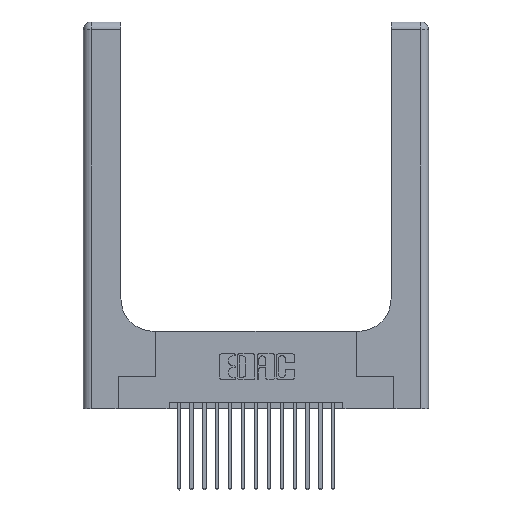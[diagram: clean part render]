
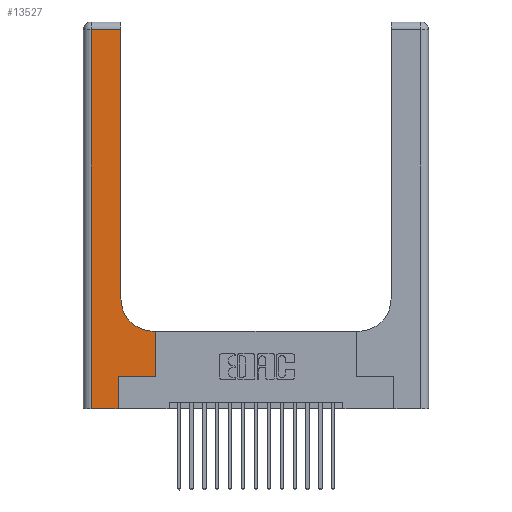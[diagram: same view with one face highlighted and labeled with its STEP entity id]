
A CAD part, top view. The second image highlights one B-rep face of the part: STEP entity #13527.
In plain terms, the highlighted planar face has unit normal (0, 0, 1).
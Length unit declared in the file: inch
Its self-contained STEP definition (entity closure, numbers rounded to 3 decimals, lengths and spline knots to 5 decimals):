
#70 = VERTEX_POINT ( 'NONE', #2962 ) ;
#95 = CARTESIAN_POINT ( 'NONE',  ( 0.06, 3., 0.37 ) ) ;
#214 = LINE ( 'NONE', #14687, #11632 ) ;
#369 = DIRECTION ( 'NONE',  ( 1., 0., 0. ) ) ;
#404 = FACE_OUTER_BOUND ( 'NONE', #9636, .T. ) ;
#464 = ORIENTED_EDGE ( 'NONE', *, *, #11493, .T. ) ;
#609 = VECTOR ( 'NONE', #3383, 39.37008 ) ;
#883 = VECTOR ( 'NONE', #18805, 39.37008 ) ;
#1662 = LINE ( 'NONE', #2473, #13062 ) ;
#1968 = EDGE_CURVE ( 'NONE', #17136, #9646, #12535, .T. ) ;
#2063 = PLANE ( 'NONE',  #4559 ) ;
#2333 = ORIENTED_EDGE ( 'NONE', *, *, #2672, .T. ) ;
#2473 = CARTESIAN_POINT ( 'NONE',  ( 0.2915, 0.6, 0.37 ) ) ;
#2625 = DIRECTION ( 'NONE',  ( 0., 1., 0. ) ) ;
#2672 = EDGE_CURVE ( 'NONE', #12663, #11301, #5974, .T. ) ;
#2962 = CARTESIAN_POINT ( 'NONE',  ( 0.06, 0., 0.37 ) ) ;
#3019 = LINE ( 'NONE', #15210, #12076 ) ;
#3383 = DIRECTION ( 'NONE',  ( 1., 0., 0. ) ) ;
#3759 = DIRECTION ( 'NONE',  ( 0., 0., -1. ) ) ;
#4023 = DIRECTION ( 'NONE',  ( -1., 0., 0. ) ) ;
#4559 = AXIS2_PLACEMENT_3D ( 'NONE', #5017, #3759, #6674 ) ;
#4581 = CARTESIAN_POINT ( 'NONE',  ( 0.269, 0., 0.37 ) ) ;
#4929 = VERTEX_POINT ( 'NONE', #9847 ) ;
#4987 = VERTEX_POINT ( 'NONE', #18731 ) ;
#5017 = CARTESIAN_POINT ( 'NONE',  ( 0., 3., 0.37 ) ) ;
#5289 = ORIENTED_EDGE ( 'NONE', *, *, #8573, .T. ) ;
#5542 = CARTESIAN_POINT ( 'NONE',  ( 0.2915, 3., 0.37 ) ) ;
#5974 = LINE ( 'NONE', #5542, #6220 ) ;
#6220 = VECTOR ( 'NONE', #13109, 39.37008 ) ;
#6235 = ORIENTED_EDGE ( 'NONE', *, *, #10613, .T. ) ;
#6674 = DIRECTION ( 'NONE',  ( -1., 0., 0. ) ) ;
#6829 = ORIENTED_EDGE ( 'NONE', *, *, #7333, .T. ) ;
#7162 = DIRECTION ( 'NONE',  ( 0., 0., -1. ) ) ;
#7333 = EDGE_CURVE ( 'NONE', #4987, #4929, #1662, .T. ) ;
#8206 = VERTEX_POINT ( 'NONE', #14205 ) ;
#8573 = EDGE_CURVE ( 'NONE', #70, #17136, #3019, .T. ) ;
#8642 = CIRCLE ( 'NONE', #11375, 0.25 ) ;
#8850 = EDGE_CURVE ( 'NONE', #9646, #8206, #16232, .T. ) ;
#8870 = CARTESIAN_POINT ( 'NONE',  ( 0.5415, 0.85, 0.37 ) ) ;
#9338 = VECTOR ( 'NONE', #11883, 39.37008 ) ;
#9636 = EDGE_LOOP ( 'NONE', ( #2333, #18656, #464, #5289, #10976, #10276, #15357, #6829, #6235 ) ) ;
#9646 = VERTEX_POINT ( 'NONE', #10710 ) ;
#9847 = CARTESIAN_POINT ( 'NONE',  ( 0.5415, 0.6, 0.37 ) ) ;
#10276 = ORIENTED_EDGE ( 'NONE', *, *, #8850, .T. ) ;
#10613 = EDGE_CURVE ( 'NONE', #4929, #12663, #8642, .T. ) ;
#10637 = CARTESIAN_POINT ( 'NONE',  ( 0.06, 2.94, 0.37 ) ) ;
#10710 = CARTESIAN_POINT ( 'NONE',  ( 0.269, 0.25, 0.37 ) ) ;
#10976 = ORIENTED_EDGE ( 'NONE', *, *, #1968, .T. ) ;
#11301 = VERTEX_POINT ( 'NONE', #18704 ) ;
#11346 = CARTESIAN_POINT ( 'NONE',  ( 0.269, 0., 0.37 ) ) ;
#11375 = AXIS2_PLACEMENT_3D ( 'NONE', #8870, #7162, #17603 ) ;
#11415 = EDGE_CURVE ( 'NONE', #11301, #17097, #214, .T. ) ;
#11493 = EDGE_CURVE ( 'NONE', #17097, #70, #11882, .T. ) ;
#11632 = VECTOR ( 'NONE', #16120, 39.37008 ) ;
#11643 = CARTESIAN_POINT ( 'NONE',  ( 0.2915, 0.85, 0.37 ) ) ;
#11882 = LINE ( 'NONE', #95, #9338 ) ;
#11883 = DIRECTION ( 'NONE',  ( 0., -1., 0. ) ) ;
#12022 = VECTOR ( 'NONE', #2625, 39.37008 ) ;
#12076 = VECTOR ( 'NONE', #369, 39.37008 ) ;
#12535 = LINE ( 'NONE', #11346, #883 ) ;
#12663 = VERTEX_POINT ( 'NONE', #11643 ) ;
#12769 = CARTESIAN_POINT ( 'NONE',  ( 0.5585, 0.25, 0.37 ) ) ;
#13062 = VECTOR ( 'NONE', #4023, 39.37008 ) ;
#13109 = DIRECTION ( 'NONE',  ( 0., 1., 0. ) ) ;
#13527 = ADVANCED_FACE ( 'NONE', ( #404 ), #2063, .F. ) ;
#14205 = CARTESIAN_POINT ( 'NONE',  ( 0.5585, 0.25, 0.37 ) ) ;
#14687 = CARTESIAN_POINT ( 'NONE',  ( 0., 2.94, 0.37 ) ) ;
#15210 = CARTESIAN_POINT ( 'NONE',  ( 0., 0., 0.37 ) ) ;
#15357 = ORIENTED_EDGE ( 'NONE', *, *, #16790, .T. ) ;
#16120 = DIRECTION ( 'NONE',  ( -1., 0., 0. ) ) ;
#16232 = LINE ( 'NONE', #16718, #609 ) ;
#16718 = CARTESIAN_POINT ( 'NONE',  ( 0.269, 0.25, 0.37 ) ) ;
#16790 = EDGE_CURVE ( 'NONE', #8206, #4987, #17651, .T. ) ;
#17097 = VERTEX_POINT ( 'NONE', #10637 ) ;
#17136 = VERTEX_POINT ( 'NONE', #4581 ) ;
#17603 = DIRECTION ( 'NONE',  ( 1., 0., 0. ) ) ;
#17651 = LINE ( 'NONE', #12769, #12022 ) ;
#18656 = ORIENTED_EDGE ( 'NONE', *, *, #11415, .T. ) ;
#18704 = CARTESIAN_POINT ( 'NONE',  ( 0.2915, 2.94, 0.37 ) ) ;
#18731 = CARTESIAN_POINT ( 'NONE',  ( 0.5585, 0.6, 0.37 ) ) ;
#18805 = DIRECTION ( 'NONE',  ( 0., 1., 0. ) ) ;
